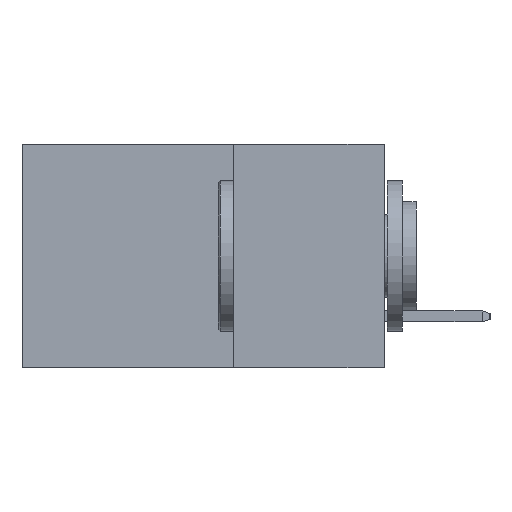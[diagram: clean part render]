
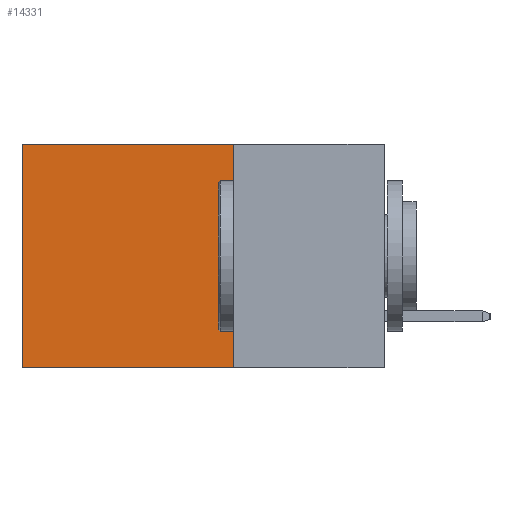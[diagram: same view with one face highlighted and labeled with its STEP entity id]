
A CAD part, left-side view. The second image highlights one B-rep face of the part: STEP entity #14331.
In plain terms, the highlighted planar face has unit normal (-1, 0, 0).
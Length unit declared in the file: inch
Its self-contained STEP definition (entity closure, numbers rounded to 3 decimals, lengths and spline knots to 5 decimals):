
#42 = DIRECTION ( 'NONE',  ( 0., 1., 0. ) ) ;
#964 = EDGE_CURVE ( 'NONE', #9831, #23169, #22441, .T. ) ;
#1734 = CARTESIAN_POINT ( 'NONE',  ( 0.2615, 0.25, -0.37 ) ) ;
#2273 = PLANE ( 'NONE',  #23105 ) ;
#2428 = CARTESIAN_POINT ( 'NONE',  ( 0.2615, 0.6, -0.37 ) ) ;
#3604 = CARTESIAN_POINT ( 'NONE',  ( 0.2615, 0.25, 0. ) ) ;
#5367 = VERTEX_POINT ( 'NONE', #22602 ) ;
#5937 = CARTESIAN_POINT ( 'NONE',  ( 0.2615, 0.25, 0. ) ) ;
#6643 = EDGE_LOOP ( 'NONE', ( #6794, #23630, #24306, #8727 ) ) ;
#6794 = ORIENTED_EDGE ( 'NONE', *, *, #16449, .T. ) ;
#7132 = VECTOR ( 'NONE', #18474, 39.37008 ) ;
#7720 = DIRECTION ( 'NONE',  ( 0., 0., -1. ) ) ;
#7861 = LINE ( 'NONE', #8508, #22558 ) ;
#8508 = CARTESIAN_POINT ( 'NONE',  ( 0.2615, 0.6, -0.37 ) ) ;
#8727 = ORIENTED_EDGE ( 'NONE', *, *, #12875, .T. ) ;
#9831 = VERTEX_POINT ( 'NONE', #18196 ) ;
#10508 = DIRECTION ( 'NONE',  ( 0., 0., -1. ) ) ;
#10991 = EDGE_CURVE ( 'NONE', #14911, #9831, #22669, .T. ) ;
#12875 = EDGE_CURVE ( 'NONE', #14911, #5367, #22598, .T. ) ;
#13563 = DIRECTION ( 'NONE',  ( 1., 0., 0. ) ) ;
#14331 = ADVANCED_FACE ( 'NONE', ( #19006 ), #2273, .F. ) ;
#14355 = CARTESIAN_POINT ( 'NONE',  ( 0.2615, 0.25, -0.37 ) ) ;
#14911 = VERTEX_POINT ( 'NONE', #3604 ) ;
#16449 = EDGE_CURVE ( 'NONE', #5367, #23169, #7861, .T. ) ;
#17090 = VECTOR ( 'NONE', #20072, 39.37008 ) ;
#17428 = CARTESIAN_POINT ( 'NONE',  ( 0.2615, 0.25, -0.37 ) ) ;
#17608 = VECTOR ( 'NONE', #42, 39.37008 ) ;
#18196 = CARTESIAN_POINT ( 'NONE',  ( 0.2615, 0.25, -0.37 ) ) ;
#18474 = DIRECTION ( 'NONE',  ( 0., 1., 0. ) ) ;
#19006 = FACE_OUTER_BOUND ( 'NONE', #6643, .T. ) ;
#20072 = DIRECTION ( 'NONE',  ( 0., 0., -1. ) ) ;
#22441 = LINE ( 'NONE', #17428, #7132 ) ;
#22558 = VECTOR ( 'NONE', #10508, 39.37008 ) ;
#22598 = LINE ( 'NONE', #5937, #17608 ) ;
#22602 = CARTESIAN_POINT ( 'NONE',  ( 0.2615, 0.6, 0. ) ) ;
#22669 = LINE ( 'NONE', #14355, #17090 ) ;
#23105 = AXIS2_PLACEMENT_3D ( 'NONE', #1734, #13563, #7720 ) ;
#23169 = VERTEX_POINT ( 'NONE', #2428 ) ;
#23630 = ORIENTED_EDGE ( 'NONE', *, *, #964, .F. ) ;
#24306 = ORIENTED_EDGE ( 'NONE', *, *, #10991, .F. ) ;
